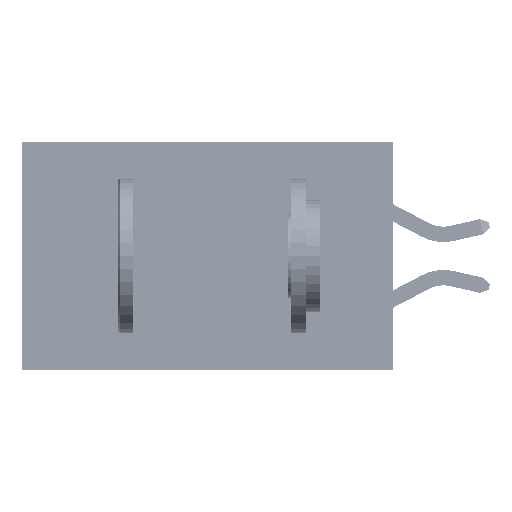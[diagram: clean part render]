
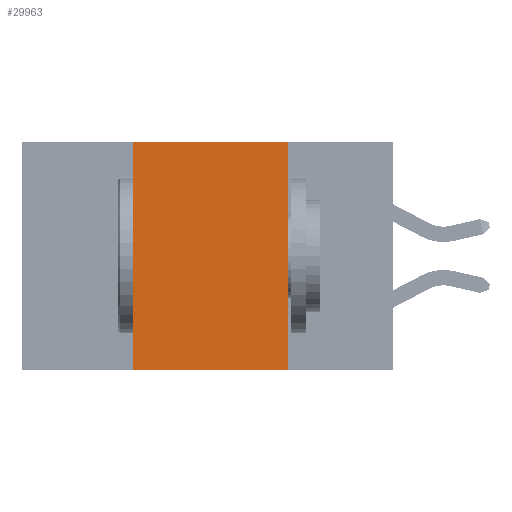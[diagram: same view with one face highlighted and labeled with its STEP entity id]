
A CAD part, left-side view. The second image highlights one B-rep face of the part: STEP entity #29963.
In plain terms, the highlighted planar face has unit normal (-1, 0, 0).
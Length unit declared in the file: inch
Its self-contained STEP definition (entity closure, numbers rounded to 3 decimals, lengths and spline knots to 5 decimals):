
#2999 = DIRECTION ( 'NONE',  ( 1., 0., 0. ) ) ;
#3070 = DIRECTION ( 'NONE',  ( 0., 0., 1. ) ) ;
#3106 = LINE ( 'NONE', #39921, #29304 ) ;
#3291 = PLANE ( 'NONE',  #37347 ) ;
#3619 = CARTESIAN_POINT ( 'NONE',  ( 0., 0.6, 0. ) ) ;
#5167 = ORIENTED_EDGE ( 'NONE', *, *, #15635, .T. ) ;
#5851 = VECTOR ( 'NONE', #41300, 39.37008 ) ;
#7312 = DIRECTION ( 'NONE',  ( 0., 0., -1. ) ) ;
#7479 = EDGE_LOOP ( 'NONE', ( #12766, #22506, #26261, #5167 ) ) ;
#7981 = EDGE_CURVE ( 'NONE', #11249, #13571, #3106, .T. ) ;
#8532 = LINE ( 'NONE', #25131, #39831 ) ;
#10293 = LINE ( 'NONE', #38382, #45504 ) ;
#11249 = VERTEX_POINT ( 'NONE', #40725 ) ;
#12766 = ORIENTED_EDGE ( 'NONE', *, *, #42967, .F. ) ;
#13571 = VERTEX_POINT ( 'NONE', #39496 ) ;
#14443 = CARTESIAN_POINT ( 'NONE',  ( 0., 0.17, -0.37 ) ) ;
#15635 = EDGE_CURVE ( 'NONE', #11249, #31277, #18373, .T. ) ;
#16641 = DIRECTION ( 'NONE',  ( 0., -1., 0. ) ) ;
#18373 = LINE ( 'NONE', #40502, #5851 ) ;
#21248 = VERTEX_POINT ( 'NONE', #30164 ) ;
#22506 = ORIENTED_EDGE ( 'NONE', *, *, #22791, .F. ) ;
#22791 = EDGE_CURVE ( 'NONE', #13571, #21248, #10293, .T. ) ;
#25131 = CARTESIAN_POINT ( 'NONE',  ( 0., 0.17, 0. ) ) ;
#26261 = ORIENTED_EDGE ( 'NONE', *, *, #7981, .F. ) ;
#29072 = DIRECTION ( 'NONE',  ( 0., 0., -1. ) ) ;
#29304 = VECTOR ( 'NONE', #3070, 39.37008 ) ;
#29686 = FACE_OUTER_BOUND ( 'NONE', #7479, .T. ) ;
#29963 = ADVANCED_FACE ( 'NONE', ( #29686 ), #3291, .F. ) ;
#30164 = CARTESIAN_POINT ( 'NONE',  ( 0., 0.17, 0. ) ) ;
#31277 = VERTEX_POINT ( 'NONE', #14443 ) ;
#37347 = AXIS2_PLACEMENT_3D ( 'NONE', #3619, #2999, #29072 ) ;
#38382 = CARTESIAN_POINT ( 'NONE',  ( 0., 0.6, 0. ) ) ;
#39496 = CARTESIAN_POINT ( 'NONE',  ( 0., 0.42, 0. ) ) ;
#39831 = VECTOR ( 'NONE', #7312, 39.37008 ) ;
#39921 = CARTESIAN_POINT ( 'NONE',  ( 0., 0.42, 0. ) ) ;
#40502 = CARTESIAN_POINT ( 'NONE',  ( 0., 0.6, -0.37 ) ) ;
#40725 = CARTESIAN_POINT ( 'NONE',  ( 0., 0.42, -0.37 ) ) ;
#41300 = DIRECTION ( 'NONE',  ( 0., -1., 0. ) ) ;
#42967 = EDGE_CURVE ( 'NONE', #21248, #31277, #8532, .T. ) ;
#45504 = VECTOR ( 'NONE', #16641, 39.37008 ) ;
